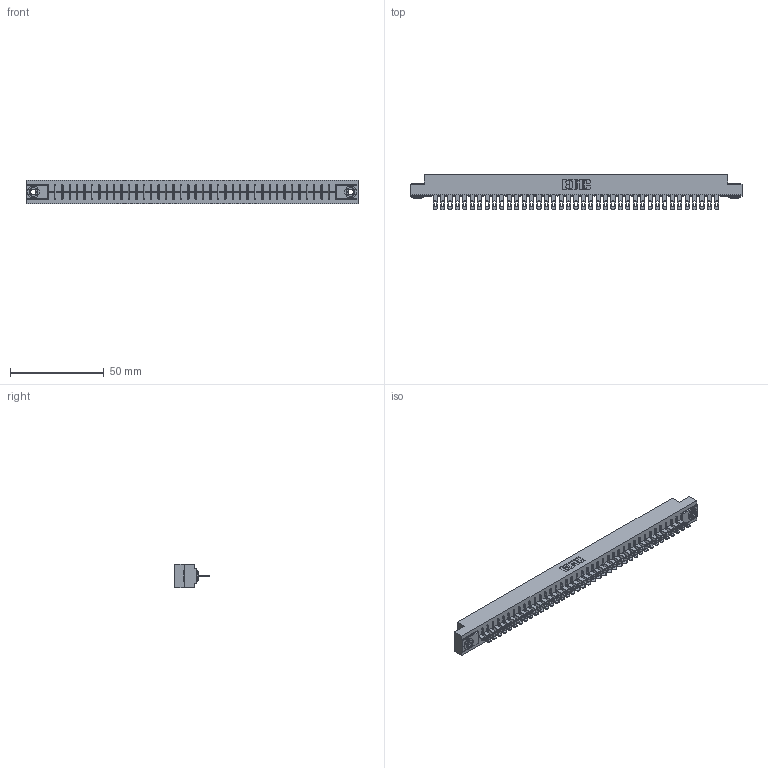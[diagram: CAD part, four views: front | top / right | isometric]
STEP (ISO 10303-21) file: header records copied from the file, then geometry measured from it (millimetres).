
FILE_DESCRIPTION (( 'STEP AP203' ), '1' );
FILE_NAME ('356-039-400-103.STEP', '2020-09-23T23:57:02', ( '' ), ( '' ), 'SwSTEP 2.0', 'SolidWorks 2020', '' );
FILE_SCHEMA (( 'CONFIG_CONTROL_DESIGN' ));
Length unit declared in the file: inch
Products named in the file (4): 306-290-001_100; 345-250-002_345-250-002-102; 356-039-400-103; 306 Part_.156 Dia
Assembly tree (42 placements, depth 2):
  356-039-400-103
    306 Part_.156 Dia
    306-290-001_100  x39
    345-250-002_345-250-002-102  x2
Bounding box: 177.55 x 18.87 x 12.7 mm (x, y, z)
Volume: 19733.5 mm3; surface area: 21166.6 mm2
Topology: 42 solids, 42 shells, 3132 faces, 8813 edges, 5662 vertices
Faces by surface type: plane 2042, cylinder 926, sphere 156, cone 8
Entity records: 37987 total; most frequent: CARTESIAN_POINT 6357, ORIENTED_EDGE 6294, DIRECTION 6283, EDGE_CURVE 3147, LINE 2451, VECTOR 2451, VERTEX_POINT 1990, AXIS2_PLACEMENT_3D 1916
